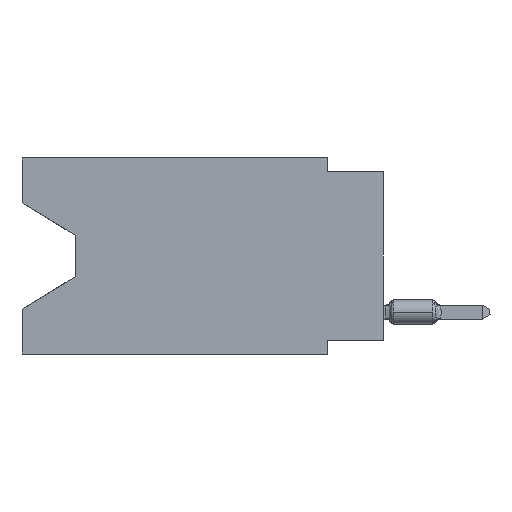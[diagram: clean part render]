
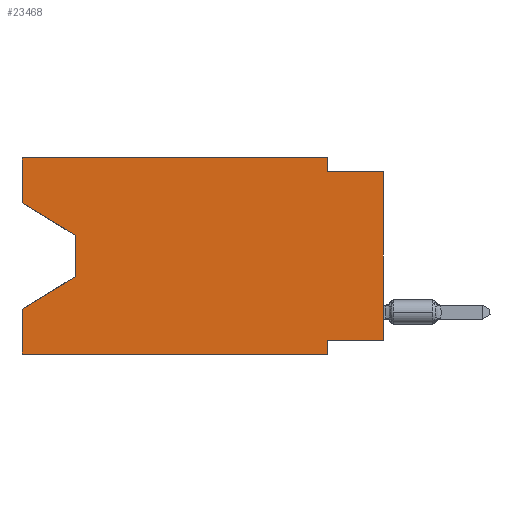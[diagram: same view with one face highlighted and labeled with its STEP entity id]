
A CAD part, left-side view. The second image highlights one B-rep face of the part: STEP entity #23468.
In plain terms, the highlighted planar face has unit normal (-1, 0, 0).
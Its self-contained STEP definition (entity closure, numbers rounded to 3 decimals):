
#113 = ORIENTED_EDGE ( 'NONE', *, *, #33211, .F. ) ;
#699 = CARTESIAN_POINT ( 'NONE',  ( 0., 13.97, -3.505 ) ) ;
#942 = CARTESIAN_POINT ( 'NONE',  ( 0., 16.383, 0. ) ) ;
#1451 = CARTESIAN_POINT ( 'NONE',  ( 0., 16.383, -2.038 ) ) ;
#1687 = CARTESIAN_POINT ( 'NONE',  ( 0., 0., -0.635 ) ) ;
#4991 = CARTESIAN_POINT ( 'NONE',  ( 0., 16.383, 0. ) ) ;
#5047 = AXIS2_PLACEMENT_3D ( 'NONE', #53807, #69243, #42935 ) ;
#6194 = EDGE_CURVE ( 'NONE', #22634, #57245, #39142, .T. ) ;
#6784 = EDGE_CURVE ( 'NONE', #42249, #56689, #30935, .T. ) ;
#7540 = DIRECTION ( 'NONE',  ( 0., 0., -1. ) ) ;
#8434 = VECTOR ( 'NONE', #57005, 1000. ) ;
#10723 = VERTEX_POINT ( 'NONE', #35631 ) ;
#10925 = ORIENTED_EDGE ( 'NONE', *, *, #6784, .F. ) ;
#13365 = ORIENTED_EDGE ( 'NONE', *, *, #53276, .T. ) ;
#14609 = VECTOR ( 'NONE', #57665, 1000. ) ;
#15115 = ORIENTED_EDGE ( 'NONE', *, *, #57917, .T. ) ;
#15674 = DIRECTION ( 'NONE',  ( 0., 1., 0. ) ) ;
#15781 = EDGE_CURVE ( 'NONE', #54521, #56689, #49296, .T. ) ;
#15911 = LINE ( 'NONE', #41176, #55506 ) ;
#17318 = CARTESIAN_POINT ( 'NONE',  ( 0., 16.383, 0. ) ) ;
#20841 = FACE_OUTER_BOUND ( 'NONE', #39388, .T. ) ;
#22091 = DIRECTION ( 'NONE',  ( 0., 0., -1. ) ) ;
#22328 = DIRECTION ( 'NONE',  ( 0., 0., 1. ) ) ;
#22580 = LINE ( 'NONE', #64345, #24293 ) ;
#22634 = VERTEX_POINT ( 'NONE', #1451 ) ;
#23468 = ADVANCED_FACE ( 'NONE', ( #20841 ), #58019, .F. ) ;
#23605 = EDGE_CURVE ( 'NONE', #46744, #10723, #36748, .T. ) ;
#23896 = EDGE_CURVE ( 'NONE', #46744, #61296, #25431, .T. ) ;
#23952 = VECTOR ( 'NONE', #22328, 1000. ) ;
#24000 = VECTOR ( 'NONE', #31996, 1000. ) ;
#24293 = VECTOR ( 'NONE', #65375, 1000. ) ;
#25431 = LINE ( 'NONE', #61928, #8434 ) ;
#25622 = CARTESIAN_POINT ( 'NONE',  ( 0., 13.97, -5.385 ) ) ;
#27136 = CARTESIAN_POINT ( 'NONE',  ( 0., 16.383, -8.89 ) ) ;
#27345 = VECTOR ( 'NONE', #32190, 1000. ) ;
#27378 = ORIENTED_EDGE ( 'NONE', *, *, #44224, .F. ) ;
#27430 = VECTOR ( 'NONE', #15674, 1000. ) ;
#27766 = VERTEX_POINT ( 'NONE', #48612 ) ;
#30796 = VECTOR ( 'NONE', #49744, 1000. ) ;
#30935 = LINE ( 'NONE', #4991, #24000 ) ;
#31996 = DIRECTION ( 'NONE',  ( 0., 0., 1. ) ) ;
#32190 = DIRECTION ( 'NONE',  ( 0., -0.855, -0.519 ) ) ;
#33211 = EDGE_CURVE ( 'NONE', #34368, #39758, #40147, .T. ) ;
#34368 = VERTEX_POINT ( 'NONE', #63477 ) ;
#35631 = CARTESIAN_POINT ( 'NONE',  ( 0., 2.54, -8.255 ) ) ;
#36748 = LINE ( 'NONE', #64100, #27430 ) ;
#37538 = LINE ( 'NONE', #699, #68957 ) ;
#37671 = LINE ( 'NONE', #27136, #14609 ) ;
#37807 = CARTESIAN_POINT ( 'NONE',  ( 0., 16.383, -2.038 ) ) ;
#39094 = CARTESIAN_POINT ( 'NONE',  ( 0., 13.97, -5.385 ) ) ;
#39142 = LINE ( 'NONE', #942, #23952 ) ;
#39388 = EDGE_LOOP ( 'NONE', ( #15115, #48956, #52875, #10925, #13365, #58982, #55961, #67624, #27378, #113, #56338, #45374 ) ) ;
#39758 = VERTEX_POINT ( 'NONE', #50767 ) ;
#39760 = CARTESIAN_POINT ( 'NONE',  ( 0., 2.54, -8.89 ) ) ;
#40147 = LINE ( 'NONE', #55953, #60641 ) ;
#41176 = CARTESIAN_POINT ( 'NONE',  ( 0., 16.383, 0. ) ) ;
#42249 = VERTEX_POINT ( 'NONE', #68646 ) ;
#42935 = DIRECTION ( 'NONE',  ( 0., 0., -1. ) ) ;
#44224 = EDGE_CURVE ( 'NONE', #39758, #61296, #65193, .T. ) ;
#44824 = EDGE_CURVE ( 'NONE', #57245, #34368, #15911, .T. ) ;
#45374 = ORIENTED_EDGE ( 'NONE', *, *, #6194, .F. ) ;
#45955 = CARTESIAN_POINT ( 'NONE',  ( 0., 0., -8.255 ) ) ;
#46196 = EDGE_CURVE ( 'NONE', #10723, #67895, #22580, .T. ) ;
#46447 = DIRECTION ( 'NONE',  ( 0., -1., 0. ) ) ;
#46744 = VERTEX_POINT ( 'NONE', #45955 ) ;
#47981 = CARTESIAN_POINT ( 'NONE',  ( 0., 16.383, -6.852 ) ) ;
#48612 = CARTESIAN_POINT ( 'NONE',  ( 0., 13.97, -3.505 ) ) ;
#48956 = ORIENTED_EDGE ( 'NONE', *, *, #59545, .T. ) ;
#49296 = LINE ( 'NONE', #39094, #51462 ) ;
#49744 = DIRECTION ( 'NONE',  ( 0., -1., 0. ) ) ;
#50767 = CARTESIAN_POINT ( 'NONE',  ( 0., 2.54, -0.635 ) ) ;
#51462 = VECTOR ( 'NONE', #59485, 1000. ) ;
#52875 = ORIENTED_EDGE ( 'NONE', *, *, #15781, .T. ) ;
#53276 = EDGE_CURVE ( 'NONE', #42249, #67895, #37671, .T. ) ;
#53807 = CARTESIAN_POINT ( 'NONE',  ( 0., 16.383, 0. ) ) ;
#54521 = VERTEX_POINT ( 'NONE', #25622 ) ;
#55506 = VECTOR ( 'NONE', #46447, 1000. ) ;
#55953 = CARTESIAN_POINT ( 'NONE',  ( 0., 2.54, 0. ) ) ;
#55961 = ORIENTED_EDGE ( 'NONE', *, *, #23605, .F. ) ;
#56338 = ORIENTED_EDGE ( 'NONE', *, *, #44824, .F. ) ;
#56689 = VERTEX_POINT ( 'NONE', #47981 ) ;
#57005 = DIRECTION ( 'NONE',  ( 0., 0., 1. ) ) ;
#57245 = VERTEX_POINT ( 'NONE', #17318 ) ;
#57665 = DIRECTION ( 'NONE',  ( 0., -1., 0. ) ) ;
#57917 = EDGE_CURVE ( 'NONE', #22634, #27766, #65152, .T. ) ;
#58019 = PLANE ( 'NONE',  #5047 ) ;
#58982 = ORIENTED_EDGE ( 'NONE', *, *, #46196, .F. ) ;
#59485 = DIRECTION ( 'NONE',  ( 0., 0.855, -0.519 ) ) ;
#59545 = EDGE_CURVE ( 'NONE', #27766, #54521, #37538, .T. ) ;
#60641 = VECTOR ( 'NONE', #7540, 1000. ) ;
#61296 = VERTEX_POINT ( 'NONE', #62290 ) ;
#61928 = CARTESIAN_POINT ( 'NONE',  ( 0., 0., 0. ) ) ;
#62290 = CARTESIAN_POINT ( 'NONE',  ( 0., 0., -0.635 ) ) ;
#63477 = CARTESIAN_POINT ( 'NONE',  ( 0., 2.54, 0. ) ) ;
#64100 = CARTESIAN_POINT ( 'NONE',  ( 0., 0., -8.255 ) ) ;
#64345 = CARTESIAN_POINT ( 'NONE',  ( 0., 2.54, -8.89 ) ) ;
#65152 = LINE ( 'NONE', #37807, #27345 ) ;
#65193 = LINE ( 'NONE', #1687, #30796 ) ;
#65375 = DIRECTION ( 'NONE',  ( 0., 0., -1. ) ) ;
#67624 = ORIENTED_EDGE ( 'NONE', *, *, #23896, .T. ) ;
#67895 = VERTEX_POINT ( 'NONE', #39760 ) ;
#68646 = CARTESIAN_POINT ( 'NONE',  ( 0., 16.383, -8.89 ) ) ;
#68957 = VECTOR ( 'NONE', #22091, 1000. ) ;
#69243 = DIRECTION ( 'NONE',  ( 1., 0., 0. ) ) ;
